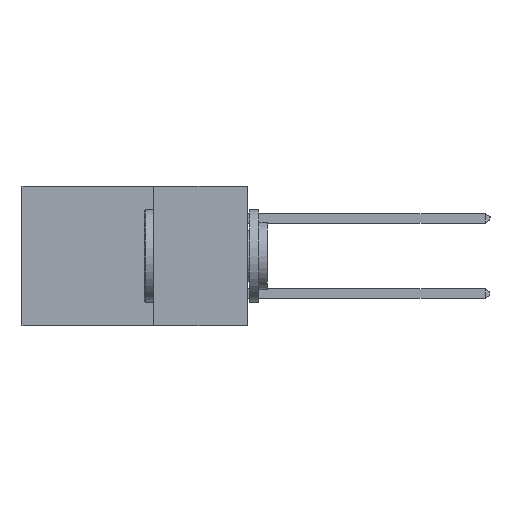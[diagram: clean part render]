
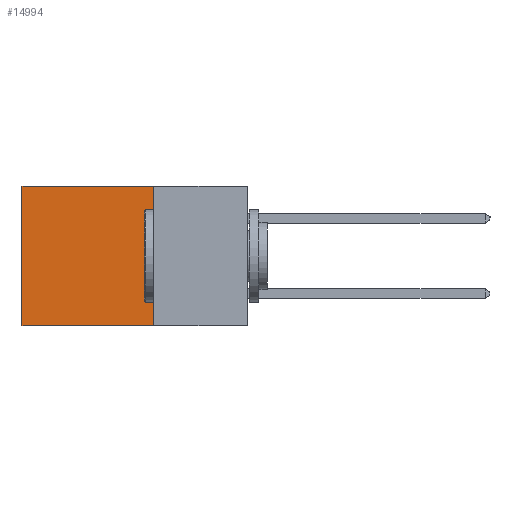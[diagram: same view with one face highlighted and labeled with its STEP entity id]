
A CAD part, left-side view. The second image highlights one B-rep face of the part: STEP entity #14994.
In plain terms, the highlighted planar face has unit normal (-1, 0, 0).
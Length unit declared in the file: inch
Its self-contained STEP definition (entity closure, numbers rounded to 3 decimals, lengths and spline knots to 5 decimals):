
#910 = LINE ( 'NONE', #7746, #6047 ) ;
#1214 = DIRECTION ( 'NONE',  ( 1., 0., 0. ) ) ;
#1615 = CARTESIAN_POINT ( 'NONE',  ( 0.2615, 0.6, -0.37 ) ) ;
#3914 = VECTOR ( 'NONE', #14886, 39.37008 ) ;
#4049 = VERTEX_POINT ( 'NONE', #1615 ) ;
#4791 = EDGE_CURVE ( 'NONE', #21606, #4049, #7733, .T. ) ;
#5408 = VERTEX_POINT ( 'NONE', #13435 ) ;
#5819 = VECTOR ( 'NONE', #6048, 39.37008 ) ;
#6047 = VECTOR ( 'NONE', #19900, 39.37008 ) ;
#6048 = DIRECTION ( 'NONE',  ( 0., 0., -1. ) ) ;
#6240 = ORIENTED_EDGE ( 'NONE', *, *, #14558, .T. ) ;
#6284 = LINE ( 'NONE', #13099, #3914 ) ;
#7032 = CARTESIAN_POINT ( 'NONE',  ( 0.2615, 0.25, 0. ) ) ;
#7733 = LINE ( 'NONE', #19447, #5819 ) ;
#7746 = CARTESIAN_POINT ( 'NONE',  ( 0.2615, 0.25, -0.37 ) ) ;
#9708 = ORIENTED_EDGE ( 'NONE', *, *, #4791, .T. ) ;
#9970 = LINE ( 'NONE', #13107, #21011 ) ;
#10852 = VERTEX_POINT ( 'NONE', #7032 ) ;
#12004 = EDGE_LOOP ( 'NONE', ( #9708, #13658, #13320, #6240 ) ) ;
#13099 = CARTESIAN_POINT ( 'NONE',  ( 0.2615, 0.25, 0. ) ) ;
#13107 = CARTESIAN_POINT ( 'NONE',  ( 0.2615, 0.25, -0.37 ) ) ;
#13320 = ORIENTED_EDGE ( 'NONE', *, *, #15900, .F. ) ;
#13435 = CARTESIAN_POINT ( 'NONE',  ( 0.2615, 0.25, -0.37 ) ) ;
#13658 = ORIENTED_EDGE ( 'NONE', *, *, #14474, .F. ) ;
#14474 = EDGE_CURVE ( 'NONE', #5408, #4049, #910, .T. ) ;
#14558 = EDGE_CURVE ( 'NONE', #10852, #21606, #6284, .T. ) ;
#14886 = DIRECTION ( 'NONE',  ( 0., 1., 0. ) ) ;
#14994 = ADVANCED_FACE ( 'NONE', ( #18305 ), #18207, .F. ) ;
#15710 = AXIS2_PLACEMENT_3D ( 'NONE', #16934, #1214, #19980 ) ;
#15900 = EDGE_CURVE ( 'NONE', #10852, #5408, #9970, .T. ) ;
#16934 = CARTESIAN_POINT ( 'NONE',  ( 0.2615, 0.25, -0.37 ) ) ;
#18207 = PLANE ( 'NONE',  #15710 ) ;
#18305 = FACE_OUTER_BOUND ( 'NONE', #12004, .T. ) ;
#19447 = CARTESIAN_POINT ( 'NONE',  ( 0.2615, 0.6, -0.37 ) ) ;
#19692 = DIRECTION ( 'NONE',  ( 0., 0., -1. ) ) ;
#19892 = CARTESIAN_POINT ( 'NONE',  ( 0.2615, 0.6, 0. ) ) ;
#19900 = DIRECTION ( 'NONE',  ( 0., 1., 0. ) ) ;
#19980 = DIRECTION ( 'NONE',  ( 0., 0., -1. ) ) ;
#21011 = VECTOR ( 'NONE', #19692, 39.37008 ) ;
#21606 = VERTEX_POINT ( 'NONE', #19892 ) ;
